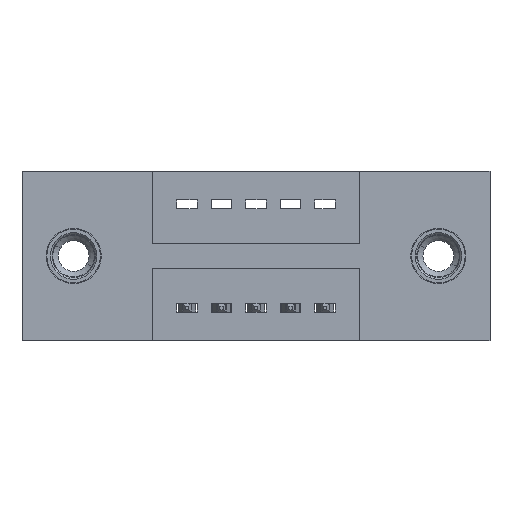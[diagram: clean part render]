
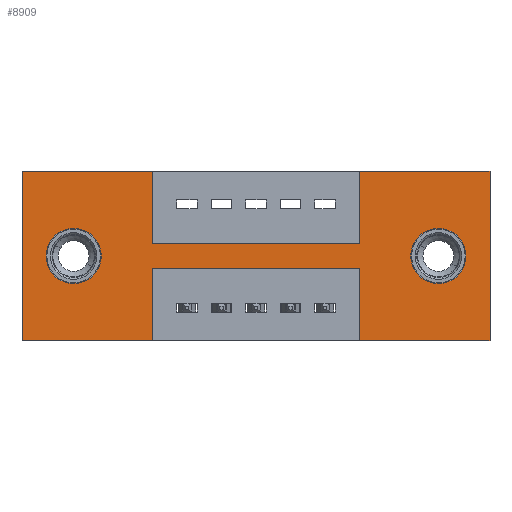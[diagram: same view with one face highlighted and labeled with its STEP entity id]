
A CAD part, front view. The second image highlights one B-rep face of the part: STEP entity #8909.
In plain terms, the highlighted planar face has unit normal (0, -1, 0).
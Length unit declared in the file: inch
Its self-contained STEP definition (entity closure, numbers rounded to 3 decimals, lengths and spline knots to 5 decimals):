
#141 = VECTOR ( 'NONE', #5862, 39.37008 ) ;
#149 = CARTESIAN_POINT ( 'NONE',  ( 0., 0., 0. ) ) ;
#171 = EDGE_CURVE ( 'NONE', #8555, #6995, #1241, .T. ) ;
#299 = VERTEX_POINT ( 'NONE', #2578 ) ;
#317 = LINE ( 'NONE', #8549, #1751 ) ;
#400 = VERTEX_POINT ( 'NONE', #3574 ) ;
#596 = CARTESIAN_POINT ( 'NONE',  ( 0., 0., -0.49 ) ) ;
#619 = DIRECTION ( 'NONE',  ( 0., -1., 0. ) ) ;
#772 = DIRECTION ( 'NONE',  ( 1., 0., 0. ) ) ;
#815 = CARTESIAN_POINT ( 'NONE',  ( 0., 0., -0.49 ) ) ;
#918 = CARTESIAN_POINT ( 'NONE',  ( 0.9775, 0., -0.28 ) ) ;
#1179 = CARTESIAN_POINT ( 'NONE',  ( 0.3775, 0., -0.49 ) ) ;
#1217 = EDGE_CURVE ( 'NONE', #8360, #4747, #1432, .T. ) ;
#1241 = LINE ( 'NONE', #6762, #5181 ) ;
#1251 = LINE ( 'NONE', #3596, #8481 ) ;
#1332 = LINE ( 'NONE', #4995, #2009 ) ;
#1345 = EDGE_CURVE ( 'NONE', #2178, #1851, #5366, .T. ) ;
#1395 = EDGE_CURVE ( 'NONE', #4295, #400, #5815, .T. ) ;
#1402 = DIRECTION ( 'NONE',  ( 0., 0., -1. ) ) ;
#1432 = LINE ( 'NONE', #149, #2763 ) ;
#1440 = VECTOR ( 'NONE', #1402, 39.37008 ) ;
#1546 = DIRECTION ( 'NONE',  ( 0., 0., -1. ) ) ;
#1560 = DIRECTION ( 'NONE',  ( 0., 0., 1. ) ) ;
#1589 = DIRECTION ( 'NONE',  ( -1., 0., 0. ) ) ;
#1705 = CARTESIAN_POINT ( 'NONE',  ( 0.9775, 0., -0.28 ) ) ;
#1751 = VECTOR ( 'NONE', #1589, 39.37008 ) ;
#1792 = DIRECTION ( 'NONE',  ( 0., 0., -1. ) ) ;
#1826 = ORIENTED_EDGE ( 'NONE', *, *, #6279, .F. ) ;
#1851 = VERTEX_POINT ( 'NONE', #2534 ) ;
#1926 = AXIS2_PLACEMENT_3D ( 'NONE', #9061, #7620, #5571 ) ;
#1949 = DIRECTION ( 'NONE',  ( 0., 0., 1. ) ) ;
#1968 = EDGE_LOOP ( 'NONE', ( #5685, #2606, #4594, #1826, #6464, #7079, #6883, #6870, #3236, #6302, #8975, #4173 ) ) ;
#2009 = VECTOR ( 'NONE', #4970, 39.37008 ) ;
#2069 = DIRECTION ( 'NONE',  ( 0., 0., -1. ) ) ;
#2096 = DIRECTION ( 'NONE',  ( 0., 1., 0. ) ) ;
#2178 = VERTEX_POINT ( 'NONE', #2610 ) ;
#2534 = CARTESIAN_POINT ( 'NONE',  ( 1.355, 0., -0.49 ) ) ;
#2578 = CARTESIAN_POINT ( 'NONE',  ( 0.3775, 0., -0.21 ) ) ;
#2580 = EDGE_CURVE ( 'NONE', #6995, #2178, #6661, .T. ) ;
#2606 = ORIENTED_EDGE ( 'NONE', *, *, #8392, .F. ) ;
#2610 = CARTESIAN_POINT ( 'NONE',  ( 1.355, 0., 0. ) ) ;
#2624 = EDGE_CURVE ( 'NONE', #4390, #7617, #5575, .T. ) ;
#2653 = VECTOR ( 'NONE', #6083, 39.37008 ) ;
#2715 = PLANE ( 'NONE',  #3270 ) ;
#2721 = VERTEX_POINT ( 'NONE', #6415 ) ;
#2741 = CARTESIAN_POINT ( 'NONE',  ( 1.2055, 0., -0.245 ) ) ;
#2763 = VECTOR ( 'NONE', #1560, 39.37008 ) ;
#2782 = EDGE_CURVE ( 'NONE', #6783, #7727, #317, .T. ) ;
#2808 = CARTESIAN_POINT ( 'NONE',  ( 1.355, 0., 0. ) ) ;
#2955 = AXIS2_PLACEMENT_3D ( 'NONE', #3722, #6505, #7205 ) ;
#2996 = VECTOR ( 'NONE', #6518, 39.37008 ) ;
#3079 = VECTOR ( 'NONE', #8539, 39.37008 ) ;
#3130 = EDGE_LOOP ( 'NONE', ( #4169, #3655 ) ) ;
#3236 = ORIENTED_EDGE ( 'NONE', *, *, #7322, .F. ) ;
#3270 = AXIS2_PLACEMENT_3D ( 'NONE', #596, #619, #2069 ) ;
#3306 = LINE ( 'NONE', #5673, #1440 ) ;
#3332 = CIRCLE ( 'NONE', #5069, 0.08 ) ;
#3404 = LINE ( 'NONE', #4966, #6362 ) ;
#3514 = VECTOR ( 'NONE', #8991, 39.37008 ) ;
#3574 = CARTESIAN_POINT ( 'NONE',  ( 1.2055, 0., -0.165 ) ) ;
#3596 = CARTESIAN_POINT ( 'NONE',  ( 0.3775, 0., -0.21 ) ) ;
#3634 = LINE ( 'NONE', #8299, #2653 ) ;
#3655 = ORIENTED_EDGE ( 'NONE', *, *, #1395, .T. ) ;
#3663 = CARTESIAN_POINT ( 'NONE',  ( 0., 0., 0. ) ) ;
#3665 = VERTEX_POINT ( 'NONE', #1179 ) ;
#3722 = CARTESIAN_POINT ( 'NONE',  ( 0.1495, 0., -0.245 ) ) ;
#3870 = CARTESIAN_POINT ( 'NONE',  ( 1.2055, 0., -0.245 ) ) ;
#3929 = EDGE_CURVE ( 'NONE', #2721, #299, #1251, .T. ) ;
#3950 = FACE_BOUND ( 'NONE', #3989, .T. ) ;
#3989 = EDGE_LOOP ( 'NONE', ( #4336, #6528 ) ) ;
#4095 = LINE ( 'NONE', #7232, #141 ) ;
#4169 = ORIENTED_EDGE ( 'NONE', *, *, #6785, .T. ) ;
#4173 = ORIENTED_EDGE ( 'NONE', *, *, #2580, .F. ) ;
#4295 = VERTEX_POINT ( 'NONE', #8896 ) ;
#4336 = ORIENTED_EDGE ( 'NONE', *, *, #6458, .T. ) ;
#4390 = VERTEX_POINT ( 'NONE', #6853 ) ;
#4557 = CARTESIAN_POINT ( 'NONE',  ( 0.9775, 0., -0.21 ) ) ;
#4594 = ORIENTED_EDGE ( 'NONE', *, *, #3929, .F. ) ;
#4661 = CARTESIAN_POINT ( 'NONE',  ( 0.9775, 0., 0. ) ) ;
#4747 = VERTEX_POINT ( 'NONE', #7988 ) ;
#4834 = LINE ( 'NONE', #918, #2996 ) ;
#4915 = DIRECTION ( 'NONE',  ( 0., 0., -1. ) ) ;
#4966 = CARTESIAN_POINT ( 'NONE',  ( 0.3775, 0., -0.21 ) ) ;
#4970 = DIRECTION ( 'NONE',  ( 1., 0., 0. ) ) ;
#4995 = CARTESIAN_POINT ( 'NONE',  ( 0., 0., 0. ) ) ;
#5070 = CARTESIAN_POINT ( 'NONE',  ( 0.9775, 0., -0.49 ) ) ;
#5069 = AXIS2_PLACEMENT_3D ( 'NONE', #3870, #8745, #1792 ) ;
#5181 = VECTOR ( 'NONE', #1949, 39.37008 ) ;
#5262 = EDGE_CURVE ( 'NONE', #3665, #8360, #4095, .T. ) ;
#5366 = LINE ( 'NONE', #2808, #3514 ) ;
#5571 = DIRECTION ( 'NONE',  ( 0., 0., 1. ) ) ;
#5575 = CIRCLE ( 'NONE', #2955, 0.08 ) ;
#5673 = CARTESIAN_POINT ( 'NONE',  ( 0.3775, 0., -0.28 ) ) ;
#5685 = ORIENTED_EDGE ( 'NONE', *, *, #171, .F. ) ;
#5740 = VERTEX_POINT ( 'NONE', #5070 ) ;
#5815 = CIRCLE ( 'NONE', #6203, 0.08 ) ;
#5862 = DIRECTION ( 'NONE',  ( -1., 0., 0. ) ) ;
#6029 = FACE_BOUND ( 'NONE', #3130, .T. ) ;
#6083 = DIRECTION ( 'NONE',  ( -1., 0., 0. ) ) ;
#6203 = AXIS2_PLACEMENT_3D ( 'NONE', #2741, #2096, #4915 ) ;
#6279 = EDGE_CURVE ( 'NONE', #4747, #2721, #1332, .T. ) ;
#6302 = ORIENTED_EDGE ( 'NONE', *, *, #7674, .F. ) ;
#6362 = VECTOR ( 'NONE', #772, 39.37008 ) ;
#6415 = CARTESIAN_POINT ( 'NONE',  ( 0.3775, 0., 0. ) ) ;
#6458 = EDGE_CURVE ( 'NONE', #7617, #4390, #6511, .T. ) ;
#6464 = ORIENTED_EDGE ( 'NONE', *, *, #1217, .F. ) ;
#6505 = DIRECTION ( 'NONE',  ( 0., 1., 0. ) ) ;
#6511 = CIRCLE ( 'NONE', #1926, 0.08 ) ;
#6518 = DIRECTION ( 'NONE',  ( 0., 0., 1. ) ) ;
#6528 = ORIENTED_EDGE ( 'NONE', *, *, #2624, .T. ) ;
#6661 = LINE ( 'NONE', #3663, #3079 ) ;
#6762 = CARTESIAN_POINT ( 'NONE',  ( 0.9775, 0., -0.21 ) ) ;
#6773 = CARTESIAN_POINT ( 'NONE',  ( 0.1495, 0., -0.165 ) ) ;
#6783 = VERTEX_POINT ( 'NONE', #1705 ) ;
#6785 = EDGE_CURVE ( 'NONE', #400, #4295, #3332, .T. ) ;
#6853 = CARTESIAN_POINT ( 'NONE',  ( 0.1495, 0., -0.325 ) ) ;
#6870 = ORIENTED_EDGE ( 'NONE', *, *, #2782, .F. ) ;
#6883 = ORIENTED_EDGE ( 'NONE', *, *, #7854, .F. ) ;
#6995 = VERTEX_POINT ( 'NONE', #4661 ) ;
#7079 = ORIENTED_EDGE ( 'NONE', *, *, #5262, .F. ) ;
#7205 = DIRECTION ( 'NONE',  ( 0., 0., 1. ) ) ;
#7232 = CARTESIAN_POINT ( 'NONE',  ( 0., 0., -0.49 ) ) ;
#7322 = EDGE_CURVE ( 'NONE', #5740, #6783, #4834, .T. ) ;
#7617 = VERTEX_POINT ( 'NONE', #6773 ) ;
#7620 = DIRECTION ( 'NONE',  ( 0., 1., 0. ) ) ;
#7674 = EDGE_CURVE ( 'NONE', #1851, #5740, #3634, .T. ) ;
#7727 = VERTEX_POINT ( 'NONE', #9041 ) ;
#7854 = EDGE_CURVE ( 'NONE', #7727, #3665, #3306, .T. ) ;
#7988 = CARTESIAN_POINT ( 'NONE',  ( 0., 0., 0. ) ) ;
#8299 = CARTESIAN_POINT ( 'NONE',  ( 0., 0., -0.49 ) ) ;
#8360 = VERTEX_POINT ( 'NONE', #815 ) ;
#8392 = EDGE_CURVE ( 'NONE', #299, #8555, #3404, .T. ) ;
#8481 = VECTOR ( 'NONE', #1546, 39.37008 ) ;
#8539 = DIRECTION ( 'NONE',  ( 1., 0., 0. ) ) ;
#8549 = CARTESIAN_POINT ( 'NONE',  ( 0.3775, 0., -0.28 ) ) ;
#8555 = VERTEX_POINT ( 'NONE', #4557 ) ;
#8745 = DIRECTION ( 'NONE',  ( 0., 1., 0. ) ) ;
#8758 = FACE_OUTER_BOUND ( 'NONE', #1968, .T. ) ;
#8896 = CARTESIAN_POINT ( 'NONE',  ( 1.2055, 0., -0.325 ) ) ;
#8909 = ADVANCED_FACE ( 'NONE', ( #6029, #3950, #8758 ), #2715, .T. ) ;
#8975 = ORIENTED_EDGE ( 'NONE', *, *, #1345, .F. ) ;
#8991 = DIRECTION ( 'NONE',  ( 0., 0., -1. ) ) ;
#9041 = CARTESIAN_POINT ( 'NONE',  ( 0.3775, 0., -0.28 ) ) ;
#9061 = CARTESIAN_POINT ( 'NONE',  ( 0.1495, 0., -0.245 ) ) ;
